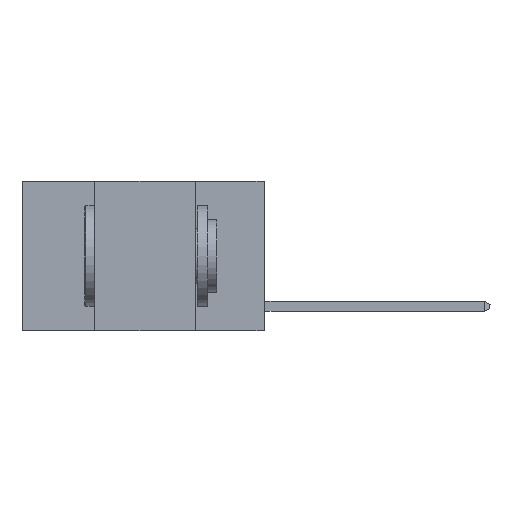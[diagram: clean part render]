
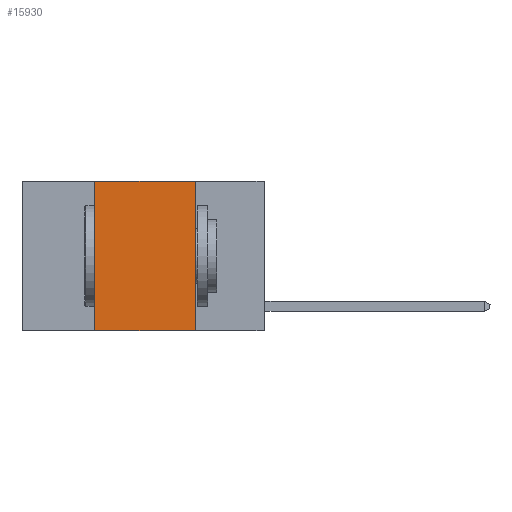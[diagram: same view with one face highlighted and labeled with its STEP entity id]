
A CAD part, left-side view. The second image highlights one B-rep face of the part: STEP entity #15930.
In plain terms, the highlighted planar face has unit normal (-1, 0, 0).
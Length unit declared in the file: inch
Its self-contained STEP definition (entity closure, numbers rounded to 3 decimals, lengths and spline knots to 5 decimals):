
#17 = VECTOR ( 'NONE', #11347, 39.37008 ) ;
#224 = CARTESIAN_POINT ( 'NONE',  ( 0., 0.17, 0. ) ) ;
#527 = CARTESIAN_POINT ( 'NONE',  ( 0., 0.6, -0.37 ) ) ;
#586 = LINE ( 'NONE', #16861, #17 ) ;
#687 = DIRECTION ( 'NONE',  ( 0., -1., 0. ) ) ;
#853 = VERTEX_POINT ( 'NONE', #16493 ) ;
#1126 = EDGE_CURVE ( 'NONE', #3762, #853, #13681, .T. ) ;
#1369 = ORIENTED_EDGE ( 'NONE', *, *, #7962, .F. ) ;
#2397 = CARTESIAN_POINT ( 'NONE',  ( 0., 0.6, 0. ) ) ;
#2456 = CARTESIAN_POINT ( 'NONE',  ( 0., 0.42, -0.37 ) ) ;
#3329 = LINE ( 'NONE', #224, #14512 ) ;
#3717 = FACE_OUTER_BOUND ( 'NONE', #11416, .T. ) ;
#3762 = VERTEX_POINT ( 'NONE', #10517 ) ;
#3828 = VERTEX_POINT ( 'NONE', #2456 ) ;
#6188 = ORIENTED_EDGE ( 'NONE', *, *, #1126, .F. ) ;
#6293 = VERTEX_POINT ( 'NONE', #7627 ) ;
#7627 = CARTESIAN_POINT ( 'NONE',  ( 0., 0.17, -0.37 ) ) ;
#7796 = DIRECTION ( 'NONE',  ( 0., 0., -1. ) ) ;
#7962 = EDGE_CURVE ( 'NONE', #3828, #3762, #586, .T. ) ;
#8912 = VECTOR ( 'NONE', #687, 39.37008 ) ;
#8929 = EDGE_CURVE ( 'NONE', #853, #6293, #3329, .T. ) ;
#8941 = VECTOR ( 'NONE', #16453, 39.37008 ) ;
#9041 = LINE ( 'NONE', #527, #8912 ) ;
#9811 = DIRECTION ( 'NONE',  ( 0., 0., -1. ) ) ;
#10517 = CARTESIAN_POINT ( 'NONE',  ( 0., 0.42, 0. ) ) ;
#11347 = DIRECTION ( 'NONE',  ( 0., 0., 1. ) ) ;
#11416 = EDGE_LOOP ( 'NONE', ( #16967, #6188, #1369, #15442 ) ) ;
#11554 = EDGE_CURVE ( 'NONE', #3828, #6293, #9041, .T. ) ;
#12919 = AXIS2_PLACEMENT_3D ( 'NONE', #2397, #15557, #7796 ) ;
#13681 = LINE ( 'NONE', #13850, #8941 ) ;
#13850 = CARTESIAN_POINT ( 'NONE',  ( 0., 0.6, 0. ) ) ;
#14512 = VECTOR ( 'NONE', #9811, 39.37008 ) ;
#14536 = PLANE ( 'NONE',  #12919 ) ;
#15442 = ORIENTED_EDGE ( 'NONE', *, *, #11554, .T. ) ;
#15557 = DIRECTION ( 'NONE',  ( 1., 0., 0. ) ) ;
#15930 = ADVANCED_FACE ( 'NONE', ( #3717 ), #14536, .F. ) ;
#16453 = DIRECTION ( 'NONE',  ( 0., -1., 0. ) ) ;
#16493 = CARTESIAN_POINT ( 'NONE',  ( 0., 0.17, 0. ) ) ;
#16861 = CARTESIAN_POINT ( 'NONE',  ( 0., 0.42, 0. ) ) ;
#16967 = ORIENTED_EDGE ( 'NONE', *, *, #8929, .F. ) ;
